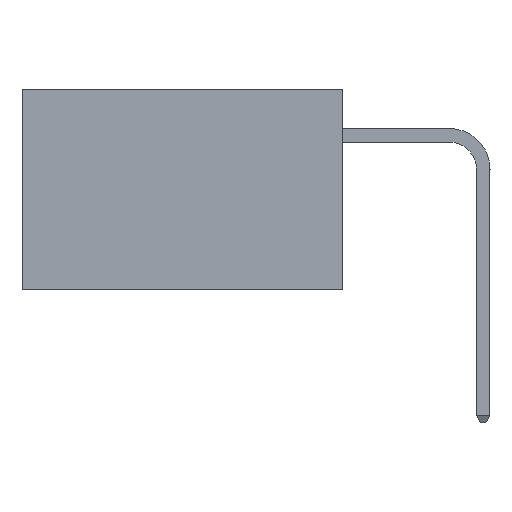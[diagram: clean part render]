
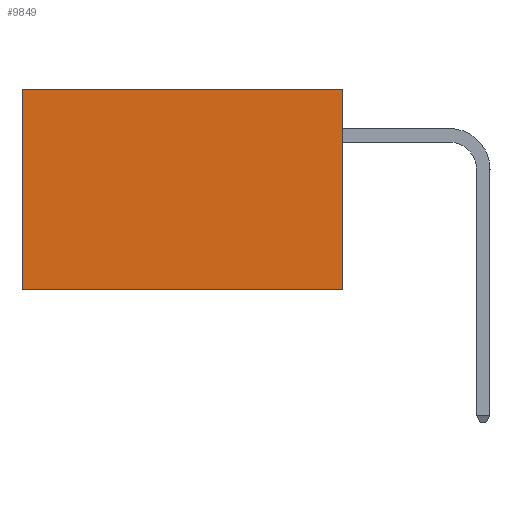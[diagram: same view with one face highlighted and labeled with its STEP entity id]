
A CAD part, left-side view. The second image highlights one B-rep face of the part: STEP entity #9849.
In plain terms, the highlighted planar face has unit normal (-1, 0, 0).
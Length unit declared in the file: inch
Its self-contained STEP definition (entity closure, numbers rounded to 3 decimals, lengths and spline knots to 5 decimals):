
#898 = EDGE_CURVE ( 'NONE', #7214, #11538, #6437, .T. ) ;
#1330 = CARTESIAN_POINT ( 'NONE',  ( 0.277, 0., -0.37 ) ) ;
#1935 = DIRECTION ( 'NONE',  ( 0., 0., -1. ) ) ;
#2211 = VERTEX_POINT ( 'NONE', #9244 ) ;
#3274 = AXIS2_PLACEMENT_3D ( 'NONE', #1330, #6907, #15959 ) ;
#3723 = LINE ( 'NONE', #4501, #16794 ) ;
#4344 = VECTOR ( 'NONE', #12778, 39.37008 ) ;
#4501 = CARTESIAN_POINT ( 'NONE',  ( 0.277, 0., -0.37 ) ) ;
#4584 = DIRECTION ( 'NONE',  ( 0., 1., 0. ) ) ;
#6437 = LINE ( 'NONE', #15383, #13063 ) ;
#6907 = DIRECTION ( 'NONE',  ( 1., 0., 0. ) ) ;
#7214 = VERTEX_POINT ( 'NONE', #15640 ) ;
#7981 = ORIENTED_EDGE ( 'NONE', *, *, #898, .T. ) ;
#8488 = EDGE_LOOP ( 'NONE', ( #7981, #16918, #16627, #13556 ) ) ;
#8531 = DIRECTION ( 'NONE',  ( 0., 0., -1. ) ) ;
#8799 = LINE ( 'NONE', #16473, #4344 ) ;
#8880 = VERTEX_POINT ( 'NONE', #15110 ) ;
#9244 = CARTESIAN_POINT ( 'NONE',  ( 0.277, 0., -0.37 ) ) ;
#9849 = ADVANCED_FACE ( 'NONE', ( #14080 ), #14712, .F. ) ;
#10048 = EDGE_CURVE ( 'NONE', #2211, #11538, #11271, .T. ) ;
#11271 = LINE ( 'NONE', #11272, #14259 ) ;
#11272 = CARTESIAN_POINT ( 'NONE',  ( 0.277, 0., -0.37 ) ) ;
#11506 = CARTESIAN_POINT ( 'NONE',  ( 0.277, 0.59, -0.37 ) ) ;
#11538 = VERTEX_POINT ( 'NONE', #11506 ) ;
#12778 = DIRECTION ( 'NONE',  ( 0., 1., 0. ) ) ;
#13063 = VECTOR ( 'NONE', #1935, 39.37008 ) ;
#13556 = ORIENTED_EDGE ( 'NONE', *, *, #15341, .T. ) ;
#14080 = FACE_OUTER_BOUND ( 'NONE', #8488, .T. ) ;
#14259 = VECTOR ( 'NONE', #4584, 39.37008 ) ;
#14712 = PLANE ( 'NONE',  #3274 ) ;
#15110 = CARTESIAN_POINT ( 'NONE',  ( 0.277, 0., 0. ) ) ;
#15208 = EDGE_CURVE ( 'NONE', #8880, #2211, #3723, .T. ) ;
#15341 = EDGE_CURVE ( 'NONE', #8880, #7214, #8799, .T. ) ;
#15383 = CARTESIAN_POINT ( 'NONE',  ( 0.277, 0.59, -0.37 ) ) ;
#15640 = CARTESIAN_POINT ( 'NONE',  ( 0.277, 0.59, 0. ) ) ;
#15959 = DIRECTION ( 'NONE',  ( 0., 0., -1. ) ) ;
#16473 = CARTESIAN_POINT ( 'NONE',  ( 0.277, 0., 0. ) ) ;
#16627 = ORIENTED_EDGE ( 'NONE', *, *, #15208, .F. ) ;
#16794 = VECTOR ( 'NONE', #8531, 39.37008 ) ;
#16918 = ORIENTED_EDGE ( 'NONE', *, *, #10048, .F. ) ;
